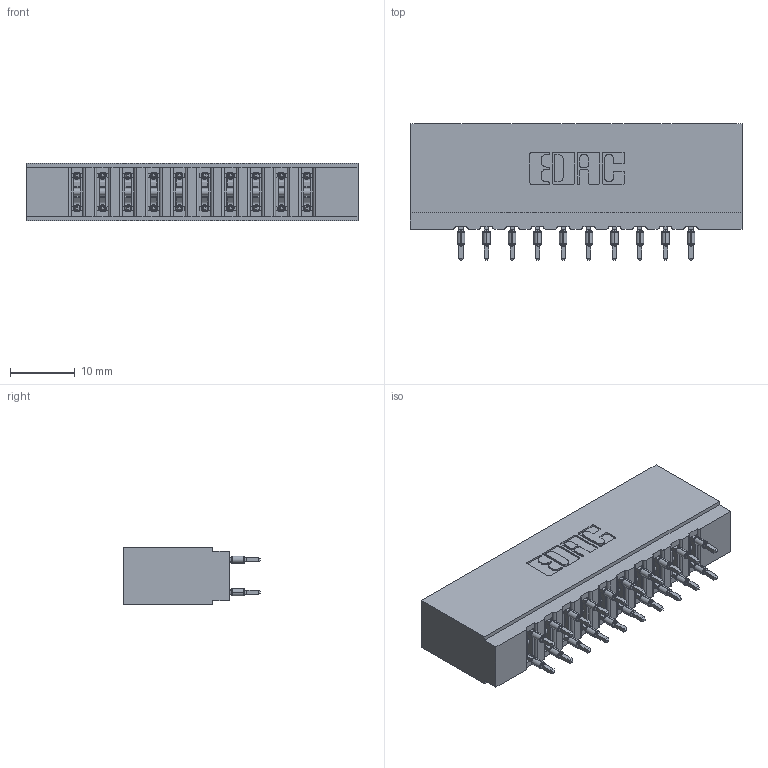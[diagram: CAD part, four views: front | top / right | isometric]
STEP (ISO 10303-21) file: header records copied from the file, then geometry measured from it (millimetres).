
FILE_DESCRIPTION (( 'STEP AP203' ), '1' );
FILE_NAME ('737-020-560-201.STEP', '2020-09-10T21:05:54', ( '' ), ( '' ), 'SwSTEP 2.0', 'SolidWorks 2020', '' );
FILE_SCHEMA (( 'CONFIG_CONTROL_DESIGN' ));
Length unit declared in the file: inch
Products named in the file (3): 737-020-560-201; 745-292-001_560; 737 Part_Insulator Option - 01
Assembly tree (21 placements, depth 2):
  737-020-560-201
    737 Part_Insulator Option - 01
    745-292-001_560  x20
Bounding box: 51.46 x 21.22 x 8.89 mm (x, y, z)
Volume: 5363.8 mm3; surface area: 7437.7 mm2
Topology: 21 solids, 21 shells, 2074 faces, 5675 edges, 3610 vertices
Faces by surface type: plane 1084, cylinder 470, bspline 400, torus 120
Entity records: 21830 total; most frequent: CARTESIAN_POINT 4303, ORIENTED_EDGE 3674, DIRECTION 3239, EDGE_CURVE 1837, VECTOR 1587, LINE 1587, VERTEX_POINT 1178, AXIS2_PLACEMENT_3D 826
